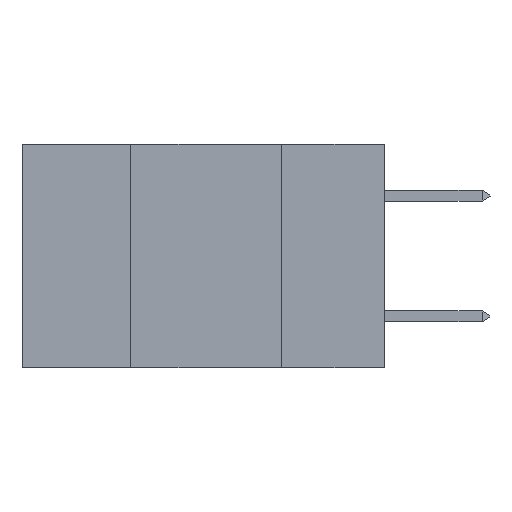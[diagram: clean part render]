
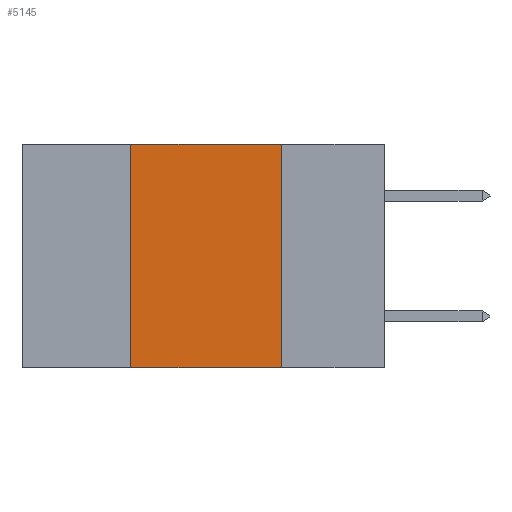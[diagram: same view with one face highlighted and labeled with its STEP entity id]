
A CAD part, left-side view. The second image highlights one B-rep face of the part: STEP entity #5145.
In plain terms, the highlighted planar face has unit normal (-1, 0, 0).
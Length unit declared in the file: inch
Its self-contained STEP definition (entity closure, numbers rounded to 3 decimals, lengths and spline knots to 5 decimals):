
#494 = EDGE_CURVE ( 'NONE', #16230, #13740, #5407, .T. ) ;
#1738 = VECTOR ( 'NONE', #13347, 39.37008 ) ;
#1929 = CARTESIAN_POINT ( 'NONE',  ( 0., 0.17, 0. ) ) ;
#2328 = DIRECTION ( 'NONE',  ( 0., 0., 1. ) ) ;
#3112 = PLANE ( 'NONE',  #5939 ) ;
#3114 = CARTESIAN_POINT ( 'NONE',  ( 0., 0.6, 0. ) ) ;
#3881 = LINE ( 'NONE', #6585, #10654 ) ;
#4317 = CARTESIAN_POINT ( 'NONE',  ( 0., 0.17, 0. ) ) ;
#5145 = ADVANCED_FACE ( 'NONE', ( #9381 ), #3112, .F. ) ;
#5307 = DIRECTION ( 'NONE',  ( 0., 0., -1. ) ) ;
#5407 = LINE ( 'NONE', #4317, #14883 ) ;
#5939 = AXIS2_PLACEMENT_3D ( 'NONE', #6659, #8102, #5307 ) ;
#6252 = VERTEX_POINT ( 'NONE', #16343 ) ;
#6585 = CARTESIAN_POINT ( 'NONE',  ( 0., 0.6, -0.37 ) ) ;
#6659 = CARTESIAN_POINT ( 'NONE',  ( 0., 0.6, 0. ) ) ;
#6815 = ORIENTED_EDGE ( 'NONE', *, *, #14557, .F. ) ;
#7182 = DIRECTION ( 'NONE',  ( 0., 0., -1. ) ) ;
#8102 = DIRECTION ( 'NONE',  ( 1., 0., 0. ) ) ;
#8152 = EDGE_CURVE ( 'NONE', #6252, #13740, #3881, .T. ) ;
#8734 = ORIENTED_EDGE ( 'NONE', *, *, #494, .F. ) ;
#9381 = FACE_OUTER_BOUND ( 'NONE', #14325, .T. ) ;
#9798 = ORIENTED_EDGE ( 'NONE', *, *, #8152, .T. ) ;
#10577 = VERTEX_POINT ( 'NONE', #15091 ) ;
#10654 = VECTOR ( 'NONE', #11742, 39.37008 ) ;
#10797 = LINE ( 'NONE', #3114, #1738 ) ;
#11742 = DIRECTION ( 'NONE',  ( 0., -1., 0. ) ) ;
#12825 = VECTOR ( 'NONE', #2328, 39.37008 ) ;
#12900 = CARTESIAN_POINT ( 'NONE',  ( 0., 0.17, -0.37 ) ) ;
#12924 = LINE ( 'NONE', #15275, #12825 ) ;
#13293 = ORIENTED_EDGE ( 'NONE', *, *, #14304, .F. ) ;
#13347 = DIRECTION ( 'NONE',  ( 0., -1., 0. ) ) ;
#13740 = VERTEX_POINT ( 'NONE', #12900 ) ;
#14304 = EDGE_CURVE ( 'NONE', #10577, #16230, #10797, .T. ) ;
#14325 = EDGE_LOOP ( 'NONE', ( #8734, #13293, #6815, #9798 ) ) ;
#14557 = EDGE_CURVE ( 'NONE', #6252, #10577, #12924, .T. ) ;
#14883 = VECTOR ( 'NONE', #7182, 39.37008 ) ;
#15091 = CARTESIAN_POINT ( 'NONE',  ( 0., 0.42, 0. ) ) ;
#15275 = CARTESIAN_POINT ( 'NONE',  ( 0., 0.42, 0. ) ) ;
#16230 = VERTEX_POINT ( 'NONE', #1929 ) ;
#16343 = CARTESIAN_POINT ( 'NONE',  ( 0., 0.42, -0.37 ) ) ;
